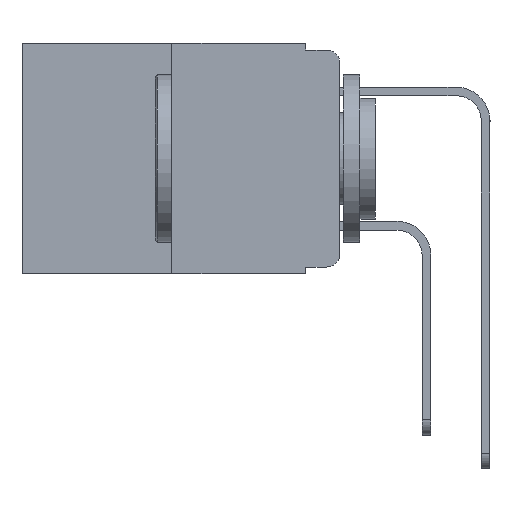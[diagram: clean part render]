
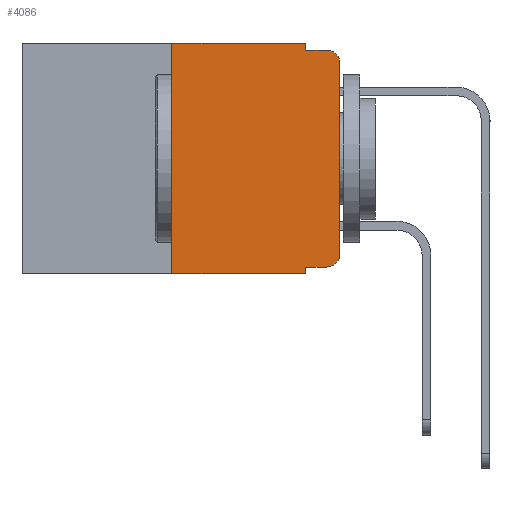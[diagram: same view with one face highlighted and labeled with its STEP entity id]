
A CAD part, left-side view. The second image highlights one B-rep face of the part: STEP entity #4086.
In plain terms, the highlighted planar face has unit normal (-1, 0, 0).
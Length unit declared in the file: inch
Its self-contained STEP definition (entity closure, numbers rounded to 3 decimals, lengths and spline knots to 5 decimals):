
#118 = CARTESIAN_POINT ( 'NONE',  ( 0., 0.051, 0. ) ) ;
#221 = CARTESIAN_POINT ( 'NONE',  ( 0., 0.051, -0.333 ) ) ;
#698 = CARTESIAN_POINT ( 'NONE',  ( 0., 0.473, -0.343 ) ) ;
#988 = LINE ( 'NONE', #5914, #6894 ) ;
#1190 = VERTEX_POINT ( 'NONE', #6085 ) ;
#1249 = CARTESIAN_POINT ( 'NONE',  ( 0., 0.051, -0.01 ) ) ;
#1255 = EDGE_CURVE ( 'NONE', #8386, #1190, #9374, .T. ) ;
#1703 = CARTESIAN_POINT ( 'NONE',  ( 0., 0.25, -0.343 ) ) ;
#1711 = LINE ( 'NONE', #7722, #13305 ) ;
#1987 = ORIENTED_EDGE ( 'NONE', *, *, #2845, .F. ) ;
#2301 = CIRCLE ( 'NONE', #8488, 0.02 ) ;
#2347 = ORIENTED_EDGE ( 'NONE', *, *, #9204, .T. ) ;
#2353 = VERTEX_POINT ( 'NONE', #221 ) ;
#2487 = CARTESIAN_POINT ( 'NONE',  ( 0., 0.25, 0. ) ) ;
#2645 = CARTESIAN_POINT ( 'NONE',  ( 0., 0., 0. ) ) ;
#2723 = ORIENTED_EDGE ( 'NONE', *, *, #13576, .T. ) ;
#2845 = EDGE_CURVE ( 'NONE', #10002, #12675, #8315, .T. ) ;
#3734 = CARTESIAN_POINT ( 'NONE',  ( 0., 0.051, 0. ) ) ;
#3935 = VERTEX_POINT ( 'NONE', #6709 ) ;
#4086 = ADVANCED_FACE ( 'NONE', ( #12519 ), #10269, .F. ) ;
#4402 = DIRECTION ( 'NONE',  ( 0., 0., 1. ) ) ;
#4560 = AXIS2_PLACEMENT_3D ( 'NONE', #12425, #5869, #13475 ) ;
#4792 = ORIENTED_EDGE ( 'NONE', *, *, #6028, .T. ) ;
#5013 = DIRECTION ( 'NONE',  ( 0., 0., 1. ) ) ;
#5094 = EDGE_LOOP ( 'NONE', ( #7494, #4792, #7844, #1987, #5163, #8186, #2347, #5524, #2723, #8875 ) ) ;
#5163 = ORIENTED_EDGE ( 'NONE', *, *, #6721, .F. ) ;
#5246 = EDGE_CURVE ( 'NONE', #12675, #3935, #1711, .T. ) ;
#5295 = VECTOR ( 'NONE', #7440, 39.37008 ) ;
#5521 = CARTESIAN_POINT ( 'NONE',  ( 0., 0.02, -0.313 ) ) ;
#5524 = ORIENTED_EDGE ( 'NONE', *, *, #14272, .F. ) ;
#5550 = DIRECTION ( 'NONE',  ( -1., 0., 0. ) ) ;
#5610 = VECTOR ( 'NONE', #5013, 39.37008 ) ;
#5869 = DIRECTION ( 'NONE',  ( 1., 0., 0. ) ) ;
#5914 = CARTESIAN_POINT ( 'NONE',  ( 0., 0.473, 0. ) ) ;
#6028 = EDGE_CURVE ( 'NONE', #13917, #3935, #2301, .T. ) ;
#6085 = CARTESIAN_POINT ( 'NONE',  ( 0., 0.25, 0. ) ) ;
#6427 = VECTOR ( 'NONE', #4402, 39.37008 ) ;
#6677 = DIRECTION ( 'NONE',  ( 0., 0., -1. ) ) ;
#6709 = CARTESIAN_POINT ( 'NONE',  ( 0., 0.02, -0.01 ) ) ;
#6721 = EDGE_CURVE ( 'NONE', #1190, #10002, #988, .T. ) ;
#6894 = VECTOR ( 'NONE', #12465, 39.37008 ) ;
#7440 = DIRECTION ( 'NONE',  ( 0., 0., -1. ) ) ;
#7494 = ORIENTED_EDGE ( 'NONE', *, *, #7554, .T. ) ;
#7554 = EDGE_CURVE ( 'NONE', #8209, #13917, #11480, .T. ) ;
#7607 = CARTESIAN_POINT ( 'NONE',  ( 0., 0.051, -0.343 ) ) ;
#7722 = CARTESIAN_POINT ( 'NONE',  ( 0., 0.051, -0.01 ) ) ;
#7844 = ORIENTED_EDGE ( 'NONE', *, *, #5246, .F. ) ;
#8047 = VECTOR ( 'NONE', #9906, 39.37008 ) ;
#8067 = CARTESIAN_POINT ( 'NONE',  ( 0., 0.051, 0. ) ) ;
#8186 = ORIENTED_EDGE ( 'NONE', *, *, #1255, .F. ) ;
#8209 = VERTEX_POINT ( 'NONE', #8329 ) ;
#8315 = LINE ( 'NONE', #118, #5295 ) ;
#8329 = CARTESIAN_POINT ( 'NONE',  ( 0., 0., -0.313 ) ) ;
#8369 = VERTEX_POINT ( 'NONE', #13920 ) ;
#8386 = VERTEX_POINT ( 'NONE', #1703 ) ;
#8488 = AXIS2_PLACEMENT_3D ( 'NONE', #12145, #5550, #13197 ) ;
#8651 = CARTESIAN_POINT ( 'NONE',  ( 0., 0.051, -0.333 ) ) ;
#8875 = ORIENTED_EDGE ( 'NONE', *, *, #12180, .T. ) ;
#9162 = DIRECTION ( 'NONE',  ( 0., 0., -1. ) ) ;
#9204 = EDGE_CURVE ( 'NONE', #8386, #9899, #10581, .T. ) ;
#9374 = LINE ( 'NONE', #2487, #6427 ) ;
#9537 = CARTESIAN_POINT ( 'NONE',  ( 0., 0., -0.03 ) ) ;
#9899 = VERTEX_POINT ( 'NONE', #7607 ) ;
#9906 = DIRECTION ( 'NONE',  ( 0., -1., 0. ) ) ;
#10002 = VERTEX_POINT ( 'NONE', #3734 ) ;
#10269 = PLANE ( 'NONE',  #4560 ) ;
#10552 = VECTOR ( 'NONE', #11895, 39.37008 ) ;
#10555 = VECTOR ( 'NONE', #9162, 39.37008 ) ;
#10581 = LINE ( 'NONE', #698, #8047 ) ;
#10700 = LINE ( 'NONE', #8067, #10555 ) ;
#11069 = AXIS2_PLACEMENT_3D ( 'NONE', #5521, #13173, #6677 ) ;
#11480 = LINE ( 'NONE', #2645, #5610 ) ;
#11895 = DIRECTION ( 'NONE',  ( 0., -1., 0. ) ) ;
#12027 = DIRECTION ( 'NONE',  ( 0., -1., 0. ) ) ;
#12145 = CARTESIAN_POINT ( 'NONE',  ( 0., 0.02, -0.03 ) ) ;
#12180 = EDGE_CURVE ( 'NONE', #8369, #8209, #13426, .T. ) ;
#12425 = CARTESIAN_POINT ( 'NONE',  ( 0., 0.473, 0. ) ) ;
#12465 = DIRECTION ( 'NONE',  ( 0., -1., 0. ) ) ;
#12519 = FACE_OUTER_BOUND ( 'NONE', #5094, .T. ) ;
#12675 = VERTEX_POINT ( 'NONE', #1249 ) ;
#13173 = DIRECTION ( 'NONE',  ( -1., 0., 0. ) ) ;
#13197 = DIRECTION ( 'NONE',  ( 0., 0., -1. ) ) ;
#13305 = VECTOR ( 'NONE', #12027, 39.37008 ) ;
#13385 = LINE ( 'NONE', #8651, #10552 ) ;
#13426 = CIRCLE ( 'NONE', #11069, 0.02 ) ;
#13475 = DIRECTION ( 'NONE',  ( 0., 0., -1. ) ) ;
#13576 = EDGE_CURVE ( 'NONE', #2353, #8369, #13385, .T. ) ;
#13917 = VERTEX_POINT ( 'NONE', #9537 ) ;
#13920 = CARTESIAN_POINT ( 'NONE',  ( 0., 0.02, -0.333 ) ) ;
#14272 = EDGE_CURVE ( 'NONE', #2353, #9899, #10700, .T. ) ;
